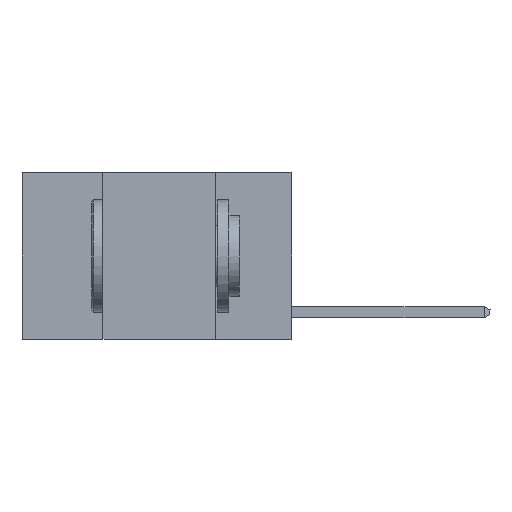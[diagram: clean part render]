
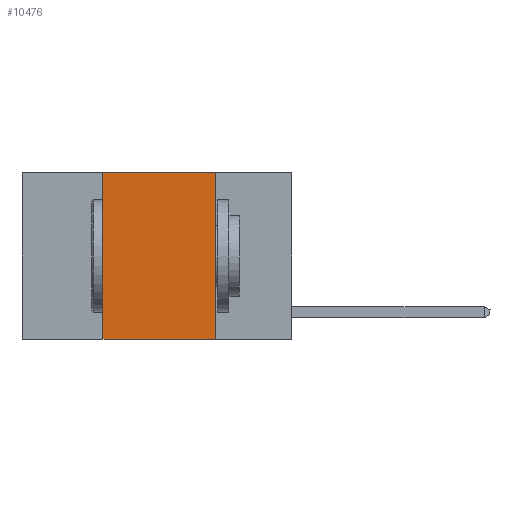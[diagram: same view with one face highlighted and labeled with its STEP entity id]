
A CAD part, left-side view. The second image highlights one B-rep face of the part: STEP entity #10476.
In plain terms, the highlighted planar face has unit normal (-1, 0, 0).
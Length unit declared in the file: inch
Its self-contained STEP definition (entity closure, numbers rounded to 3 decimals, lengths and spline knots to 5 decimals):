
#299 = VECTOR ( 'NONE', #7601, 39.37008 ) ;
#1119 = DIRECTION ( 'NONE',  ( 0., -1., 0. ) ) ;
#1308 = EDGE_CURVE ( 'NONE', #4804, #15399, #12760, .T. ) ;
#1574 = CARTESIAN_POINT ( 'NONE',  ( 0., 0.17, -0.37 ) ) ;
#1683 = ORIENTED_EDGE ( 'NONE', *, *, #1308, .F. ) ;
#2203 = CARTESIAN_POINT ( 'NONE',  ( 0., 0.17, 0. ) ) ;
#2453 = PLANE ( 'NONE',  #9627 ) ;
#2790 = VECTOR ( 'NONE', #13661, 39.37008 ) ;
#3114 = ORIENTED_EDGE ( 'NONE', *, *, #22296, .F. ) ;
#3291 = DIRECTION ( 'NONE',  ( 0., 0., 1. ) ) ;
#4804 = VERTEX_POINT ( 'NONE', #2203 ) ;
#4942 = CARTESIAN_POINT ( 'NONE',  ( 0., 0.17, 0. ) ) ;
#5029 = VERTEX_POINT ( 'NONE', #20345 ) ;
#5710 = LINE ( 'NONE', #8025, #14631 ) ;
#7379 = LINE ( 'NONE', #8522, #18785 ) ;
#7601 = DIRECTION ( 'NONE',  ( 0., -1., 0. ) ) ;
#7656 = EDGE_CURVE ( 'NONE', #5029, #15399, #5710, .T. ) ;
#8025 = CARTESIAN_POINT ( 'NONE',  ( 0., 0.6, -0.37 ) ) ;
#8522 = CARTESIAN_POINT ( 'NONE',  ( 0., 0.42, 0. ) ) ;
#9627 = AXIS2_PLACEMENT_3D ( 'NONE', #18441, #22288, #13401 ) ;
#10098 = VERTEX_POINT ( 'NONE', #22807 ) ;
#10476 = ADVANCED_FACE ( 'NONE', ( #13155 ), #2453, .F. ) ;
#12760 = LINE ( 'NONE', #4942, #2790 ) ;
#13155 = FACE_OUTER_BOUND ( 'NONE', #22558, .T. ) ;
#13401 = DIRECTION ( 'NONE',  ( 0., 0., -1. ) ) ;
#13661 = DIRECTION ( 'NONE',  ( 0., 0., -1. ) ) ;
#14078 = EDGE_CURVE ( 'NONE', #10098, #4804, #17206, .T. ) ;
#14631 = VECTOR ( 'NONE', #1119, 39.37008 ) ;
#15225 = ORIENTED_EDGE ( 'NONE', *, *, #14078, .F. ) ;
#15399 = VERTEX_POINT ( 'NONE', #1574 ) ;
#17206 = LINE ( 'NONE', #18482, #299 ) ;
#18441 = CARTESIAN_POINT ( 'NONE',  ( 0., 0.6, 0. ) ) ;
#18482 = CARTESIAN_POINT ( 'NONE',  ( 0., 0.6, 0. ) ) ;
#18785 = VECTOR ( 'NONE', #3291, 39.37008 ) ;
#19368 = ORIENTED_EDGE ( 'NONE', *, *, #7656, .T. ) ;
#20345 = CARTESIAN_POINT ( 'NONE',  ( 0., 0.42, -0.37 ) ) ;
#22288 = DIRECTION ( 'NONE',  ( 1., 0., 0. ) ) ;
#22296 = EDGE_CURVE ( 'NONE', #5029, #10098, #7379, .T. ) ;
#22558 = EDGE_LOOP ( 'NONE', ( #1683, #15225, #3114, #19368 ) ) ;
#22807 = CARTESIAN_POINT ( 'NONE',  ( 0., 0.42, 0. ) ) ;
